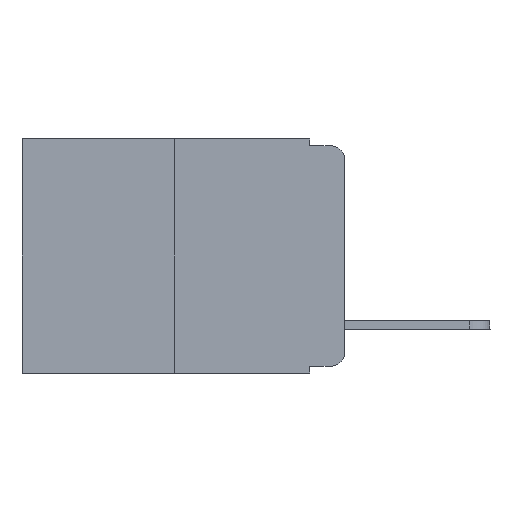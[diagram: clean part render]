
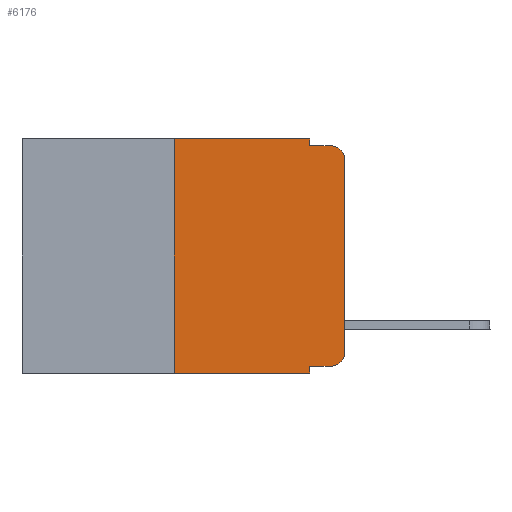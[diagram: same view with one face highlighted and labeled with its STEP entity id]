
A CAD part, left-side view. The second image highlights one B-rep face of the part: STEP entity #6176.
In plain terms, the highlighted planar face has unit normal (-1, 0, 0).
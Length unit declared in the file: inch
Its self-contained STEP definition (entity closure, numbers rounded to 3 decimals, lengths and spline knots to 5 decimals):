
#33 = VERTEX_POINT ( 'NONE', #6294 ) ;
#49 = VERTEX_POINT ( 'NONE', #6021 ) ;
#78 = VECTOR ( 'NONE', #8663, 39.37008 ) ;
#110 = EDGE_CURVE ( 'NONE', #6804, #12082, #12110, .T. ) ;
#304 = CARTESIAN_POINT ( 'NONE',  ( 0., 0.25, 0. ) ) ;
#456 = VERTEX_POINT ( 'NONE', #7364 ) ;
#584 = DIRECTION ( 'NONE',  ( 0., -1., 0. ) ) ;
#827 = DIRECTION ( 'NONE',  ( -1., 0., 0. ) ) ;
#882 = CARTESIAN_POINT ( 'NONE',  ( 0., 0.25, 0. ) ) ;
#1081 = LINE ( 'NONE', #3141, #5619 ) ;
#1150 = VECTOR ( 'NONE', #8662, 39.37008 ) ;
#1289 = EDGE_CURVE ( 'NONE', #8100, #49, #1081, .T. ) ;
#1374 = DIRECTION ( 'NONE',  ( 0., 0., -1. ) ) ;
#1573 = FACE_OUTER_BOUND ( 'NONE', #5325, .T. ) ;
#1655 = CARTESIAN_POINT ( 'NONE',  ( 0., 0.473, 0. ) ) ;
#1987 = EDGE_CURVE ( 'NONE', #5869, #456, #3953, .T. ) ;
#2008 = VECTOR ( 'NONE', #4318, 39.37008 ) ;
#2454 = LINE ( 'NONE', #1655, #3747 ) ;
#2498 = ORIENTED_EDGE ( 'NONE', *, *, #5009, .T. ) ;
#2520 = AXIS2_PLACEMENT_3D ( 'NONE', #7212, #3288, #1374 ) ;
#2550 = AXIS2_PLACEMENT_3D ( 'NONE', #9573, #12594, #7623 ) ;
#3041 = LINE ( 'NONE', #5140, #7659 ) ;
#3141 = CARTESIAN_POINT ( 'NONE',  ( 0., 0.051, -0.01 ) ) ;
#3285 = LINE ( 'NONE', #304, #2008 ) ;
#3288 = DIRECTION ( 'NONE',  ( -1., 0., 0. ) ) ;
#3299 = EDGE_CURVE ( 'NONE', #3472, #8100, #3041, .T. ) ;
#3472 = VERTEX_POINT ( 'NONE', #5349 ) ;
#3534 = VECTOR ( 'NONE', #3626, 39.37008 ) ;
#3626 = DIRECTION ( 'NONE',  ( 0., 0., -1. ) ) ;
#3729 = VERTEX_POINT ( 'NONE', #5523 ) ;
#3747 = VECTOR ( 'NONE', #584, 39.37008 ) ;
#3953 = CIRCLE ( 'NONE', #2520, 0.02 ) ;
#4180 = AXIS2_PLACEMENT_3D ( 'NONE', #7010, #827, #6816 ) ;
#4193 = CARTESIAN_POINT ( 'NONE',  ( 0., 0.02, -0.333 ) ) ;
#4318 = DIRECTION ( 'NONE',  ( 0., 0., 1. ) ) ;
#4409 = VECTOR ( 'NONE', #9227, 39.37008 ) ;
#5009 = EDGE_CURVE ( 'NONE', #33, #5869, #11035, .T. ) ;
#5140 = CARTESIAN_POINT ( 'NONE',  ( 0., 0.051, 0. ) ) ;
#5252 = CARTESIAN_POINT ( 'NONE',  ( 0., 0.473, -0.343 ) ) ;
#5325 = EDGE_LOOP ( 'NONE', ( #10822, #7890, #12025, #12157, #8155, #9915, #5472, #9509, #2498, #9974 ) ) ;
#5349 = CARTESIAN_POINT ( 'NONE',  ( 0., 0.051, 0. ) ) ;
#5472 = ORIENTED_EDGE ( 'NONE', *, *, #110, .T. ) ;
#5523 = CARTESIAN_POINT ( 'NONE',  ( 0., 0., -0.03 ) ) ;
#5587 = PLANE ( 'NONE',  #2550 ) ;
#5606 = CARTESIAN_POINT ( 'NONE',  ( 0., 0.051, 0. ) ) ;
#5619 = VECTOR ( 'NONE', #12043, 39.37008 ) ;
#5869 = VERTEX_POINT ( 'NONE', #4193 ) ;
#6021 = CARTESIAN_POINT ( 'NONE',  ( 0., 0.02, -0.01 ) ) ;
#6176 = ADVANCED_FACE ( 'NONE', ( #1573 ), #5587, .F. ) ;
#6214 = VERTEX_POINT ( 'NONE', #882 ) ;
#6290 = CIRCLE ( 'NONE', #4180, 0.02 ) ;
#6294 = CARTESIAN_POINT ( 'NONE',  ( 0., 0.051, -0.333 ) ) ;
#6632 = LINE ( 'NONE', #10547, #1150 ) ;
#6804 = VERTEX_POINT ( 'NONE', #11180 ) ;
#6816 = DIRECTION ( 'NONE',  ( 0., 0., -1. ) ) ;
#7010 = CARTESIAN_POINT ( 'NONE',  ( 0., 0.02, -0.03 ) ) ;
#7212 = CARTESIAN_POINT ( 'NONE',  ( 0., 0.02, -0.313 ) ) ;
#7364 = CARTESIAN_POINT ( 'NONE',  ( 0., 0., -0.313 ) ) ;
#7603 = CARTESIAN_POINT ( 'NONE',  ( 0., 0.051, -0.01 ) ) ;
#7623 = DIRECTION ( 'NONE',  ( 0., 0., -1. ) ) ;
#7659 = VECTOR ( 'NONE', #9971, 39.37008 ) ;
#7890 = ORIENTED_EDGE ( 'NONE', *, *, #12868, .T. ) ;
#8100 = VERTEX_POINT ( 'NONE', #7603 ) ;
#8155 = ORIENTED_EDGE ( 'NONE', *, *, #11399, .F. ) ;
#8662 = DIRECTION ( 'NONE',  ( 0., 0., 1. ) ) ;
#8663 = DIRECTION ( 'NONE',  ( 0., -1., 0. ) ) ;
#8841 = EDGE_CURVE ( 'NONE', #6804, #6214, #3285, .T. ) ;
#8902 = EDGE_CURVE ( 'NONE', #456, #3729, #6632, .T. ) ;
#9227 = DIRECTION ( 'NONE',  ( 0., -1., 0. ) ) ;
#9391 = LINE ( 'NONE', #5606, #3534 ) ;
#9509 = ORIENTED_EDGE ( 'NONE', *, *, #11414, .F. ) ;
#9573 = CARTESIAN_POINT ( 'NONE',  ( 0., 0.473, 0. ) ) ;
#9915 = ORIENTED_EDGE ( 'NONE', *, *, #8841, .F. ) ;
#9971 = DIRECTION ( 'NONE',  ( 0., 0., -1. ) ) ;
#9974 = ORIENTED_EDGE ( 'NONE', *, *, #1987, .T. ) ;
#10547 = CARTESIAN_POINT ( 'NONE',  ( 0., 0., 0. ) ) ;
#10822 = ORIENTED_EDGE ( 'NONE', *, *, #8902, .T. ) ;
#11022 = CARTESIAN_POINT ( 'NONE',  ( 0., 0.051, -0.343 ) ) ;
#11035 = LINE ( 'NONE', #11740, #78 ) ;
#11180 = CARTESIAN_POINT ( 'NONE',  ( 0., 0.25, -0.343 ) ) ;
#11399 = EDGE_CURVE ( 'NONE', #6214, #3472, #2454, .T. ) ;
#11414 = EDGE_CURVE ( 'NONE', #33, #12082, #9391, .T. ) ;
#11740 = CARTESIAN_POINT ( 'NONE',  ( 0., 0.051, -0.333 ) ) ;
#12025 = ORIENTED_EDGE ( 'NONE', *, *, #1289, .F. ) ;
#12043 = DIRECTION ( 'NONE',  ( 0., -1., 0. ) ) ;
#12082 = VERTEX_POINT ( 'NONE', #11022 ) ;
#12110 = LINE ( 'NONE', #5252, #4409 ) ;
#12157 = ORIENTED_EDGE ( 'NONE', *, *, #3299, .F. ) ;
#12594 = DIRECTION ( 'NONE',  ( 1., 0., 0. ) ) ;
#12868 = EDGE_CURVE ( 'NONE', #3729, #49, #6290, .T. ) ;
